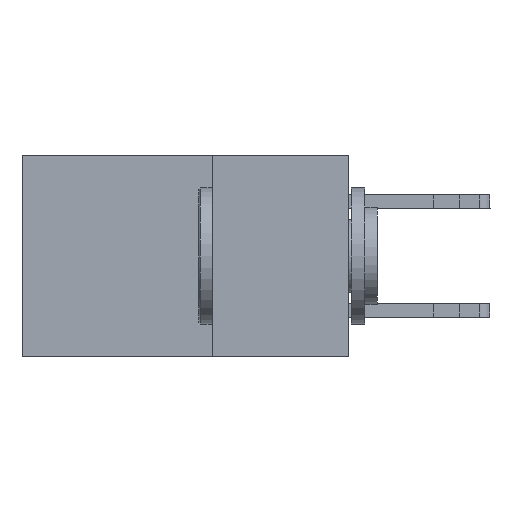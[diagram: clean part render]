
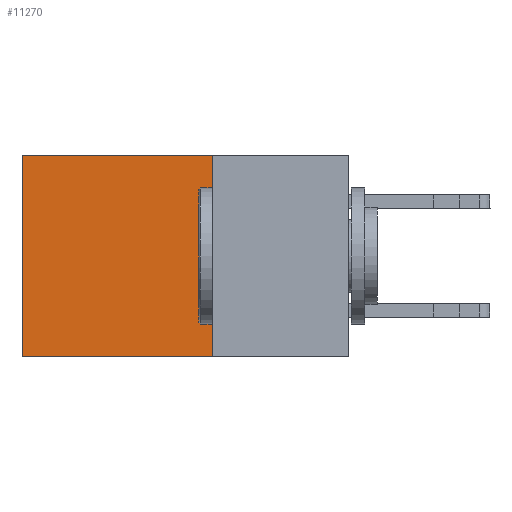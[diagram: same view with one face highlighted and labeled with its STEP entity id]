
A CAD part, left-side view. The second image highlights one B-rep face of the part: STEP entity #11270.
In plain terms, the highlighted planar face has unit normal (-1, 0, 0).
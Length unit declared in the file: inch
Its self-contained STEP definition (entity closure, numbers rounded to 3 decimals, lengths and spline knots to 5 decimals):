
#115 = EDGE_CURVE ( 'NONE', #7377, #230, #14419, .T. ) ;
#230 = VERTEX_POINT ( 'NONE', #2197 ) ;
#816 = CARTESIAN_POINT ( 'NONE',  ( 0.2615, 0.25, -0.37 ) ) ;
#2197 = CARTESIAN_POINT ( 'NONE',  ( 0.2615, 0.6, -0.37 ) ) ;
#2461 = AXIS2_PLACEMENT_3D ( 'NONE', #5938, #14111, #12411 ) ;
#3197 = CARTESIAN_POINT ( 'NONE',  ( 0.2615, 0.25, 0. ) ) ;
#4056 = VECTOR ( 'NONE', #6286, 39.37008 ) ;
#4133 = PLANE ( 'NONE',  #2461 ) ;
#4288 = EDGE_LOOP ( 'NONE', ( #10138, #20032, #18585, #16391 ) ) ;
#4311 = VECTOR ( 'NONE', #5567, 39.37008 ) ;
#4914 = VERTEX_POINT ( 'NONE', #16695 ) ;
#5567 = DIRECTION ( 'NONE',  ( 0., 0., -1. ) ) ;
#5938 = CARTESIAN_POINT ( 'NONE',  ( 0.2615, 0.25, -0.37 ) ) ;
#5955 = EDGE_CURVE ( 'NONE', #17049, #230, #11090, .T. ) ;
#6286 = DIRECTION ( 'NONE',  ( 0., 0., -1. ) ) ;
#7377 = VERTEX_POINT ( 'NONE', #14740 ) ;
#8066 = VECTOR ( 'NONE', #17767, 39.37008 ) ;
#9387 = CARTESIAN_POINT ( 'NONE',  ( 0.2615, 0.25, -0.37 ) ) ;
#9667 = DIRECTION ( 'NONE',  ( 0., 1., 0. ) ) ;
#10138 = ORIENTED_EDGE ( 'NONE', *, *, #115, .T. ) ;
#11090 = LINE ( 'NONE', #9387, #8066 ) ;
#11270 = ADVANCED_FACE ( 'NONE', ( #18672 ), #4133, .F. ) ;
#12411 = DIRECTION ( 'NONE',  ( 0., 0., -1. ) ) ;
#13639 = CARTESIAN_POINT ( 'NONE',  ( 0.2615, 0.25, -0.37 ) ) ;
#14054 = VECTOR ( 'NONE', #9667, 39.37008 ) ;
#14111 = DIRECTION ( 'NONE',  ( 1., 0., 0. ) ) ;
#14419 = LINE ( 'NONE', #14525, #4056 ) ;
#14525 = CARTESIAN_POINT ( 'NONE',  ( 0.2615, 0.6, -0.37 ) ) ;
#14740 = CARTESIAN_POINT ( 'NONE',  ( 0.2615, 0.6, 0. ) ) ;
#15081 = EDGE_CURVE ( 'NONE', #4914, #7377, #17724, .T. ) ;
#15331 = LINE ( 'NONE', #13639, #4311 ) ;
#16391 = ORIENTED_EDGE ( 'NONE', *, *, #15081, .T. ) ;
#16695 = CARTESIAN_POINT ( 'NONE',  ( 0.2615, 0.25, 0. ) ) ;
#17049 = VERTEX_POINT ( 'NONE', #816 ) ;
#17466 = EDGE_CURVE ( 'NONE', #4914, #17049, #15331, .T. ) ;
#17724 = LINE ( 'NONE', #3197, #14054 ) ;
#17767 = DIRECTION ( 'NONE',  ( 0., 1., 0. ) ) ;
#18585 = ORIENTED_EDGE ( 'NONE', *, *, #17466, .F. ) ;
#18672 = FACE_OUTER_BOUND ( 'NONE', #4288, .T. ) ;
#20032 = ORIENTED_EDGE ( 'NONE', *, *, #5955, .F. ) ;
